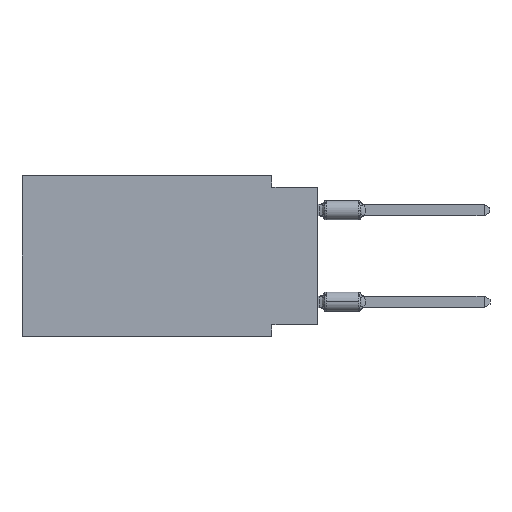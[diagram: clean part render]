
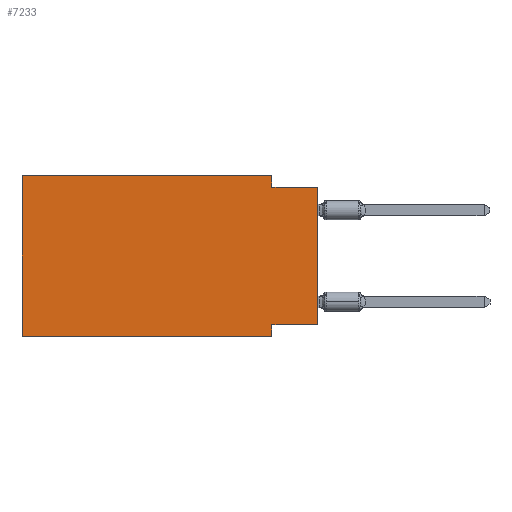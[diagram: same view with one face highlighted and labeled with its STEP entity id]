
A CAD part, left-side view. The second image highlights one B-rep face of the part: STEP entity #7233.
In plain terms, the highlighted planar face has unit normal (-1, 0, 0).
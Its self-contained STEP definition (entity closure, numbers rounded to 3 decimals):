
#296 = LINE ( 'NONE', #4620, #5544 ) ;
#353 = VECTOR ( 'NONE', #8296, 1000. ) ;
#519 = DIRECTION ( 'NONE',  ( 0., 0., -1. ) ) ;
#1118 = VECTOR ( 'NONE', #7778, 1000. ) ;
#1343 = CARTESIAN_POINT ( 'NONE',  ( 0., 16.383, 0. ) ) ;
#1543 = LINE ( 'NONE', #9942, #6392 ) ;
#2007 = VERTEX_POINT ( 'NONE', #5867 ) ;
#2042 = VECTOR ( 'NONE', #11174, 1000. ) ;
#2226 = LINE ( 'NONE', #13601, #12030 ) ;
#2514 = CARTESIAN_POINT ( 'NONE',  ( 0., 2.54, 0. ) ) ;
#2855 = LINE ( 'NONE', #3956, #353 ) ;
#3309 = EDGE_CURVE ( 'NONE', #2007, #12671, #7925, .T. ) ;
#3340 = CARTESIAN_POINT ( 'NONE',  ( 0., 0., -0.635 ) ) ;
#3508 = CARTESIAN_POINT ( 'NONE',  ( 0., 16.383, 0. ) ) ;
#3920 = ORIENTED_EDGE ( 'NONE', *, *, #8619, .F. ) ;
#3956 = CARTESIAN_POINT ( 'NONE',  ( 0., 2.54, 0. ) ) ;
#4610 = DIRECTION ( 'NONE',  ( 0., 0., 1. ) ) ;
#4620 = CARTESIAN_POINT ( 'NONE',  ( 0., 16.383, 0. ) ) ;
#4792 = EDGE_CURVE ( 'NONE', #8683, #11143, #296, .T. ) ;
#5430 = VERTEX_POINT ( 'NONE', #5609 ) ;
#5544 = VECTOR ( 'NONE', #12830, 1000. ) ;
#5609 = CARTESIAN_POINT ( 'NONE',  ( 0., 2.54, -8.255 ) ) ;
#5702 = LINE ( 'NONE', #3508, #5746 ) ;
#5746 = VECTOR ( 'NONE', #4610, 1000. ) ;
#5867 = CARTESIAN_POINT ( 'NONE',  ( 0., 0., -8.255 ) ) ;
#5999 = VERTEX_POINT ( 'NONE', #11868 ) ;
#6045 = ORIENTED_EDGE ( 'NONE', *, *, #11906, .F. ) ;
#6241 = ORIENTED_EDGE ( 'NONE', *, *, #3309, .T. ) ;
#6392 = VECTOR ( 'NONE', #519, 1000. ) ;
#6410 = DIRECTION ( 'NONE',  ( 0., 1., 0. ) ) ;
#6946 = EDGE_CURVE ( 'NONE', #11143, #5999, #2855, .T. ) ;
#7233 = ADVANCED_FACE ( 'NONE', ( #10013 ), #7601, .F. ) ;
#7494 = CARTESIAN_POINT ( 'NONE',  ( 0., 16.383, -8.89 ) ) ;
#7601 = PLANE ( 'NONE',  #8258 ) ;
#7654 = CARTESIAN_POINT ( 'NONE',  ( 0., 16.383, 0. ) ) ;
#7778 = DIRECTION ( 'NONE',  ( 0., -1., 0. ) ) ;
#7925 = LINE ( 'NONE', #12210, #2042 ) ;
#7982 = CARTESIAN_POINT ( 'NONE',  ( 0., 0., -0.635 ) ) ;
#8111 = DIRECTION ( 'NONE',  ( 0., -1., 0. ) ) ;
#8258 = AXIS2_PLACEMENT_3D ( 'NONE', #1343, #9876, #10774 ) ;
#8296 = DIRECTION ( 'NONE',  ( 0., 0., -1. ) ) ;
#8545 = CARTESIAN_POINT ( 'NONE',  ( 0., 2.54, -8.89 ) ) ;
#8619 = EDGE_CURVE ( 'NONE', #2007, #5430, #2226, .T. ) ;
#8683 = VERTEX_POINT ( 'NONE', #7654 ) ;
#9019 = ORIENTED_EDGE ( 'NONE', *, *, #11236, .F. ) ;
#9079 = VECTOR ( 'NONE', #8111, 1000. ) ;
#9876 = DIRECTION ( 'NONE',  ( 1., 0., 0. ) ) ;
#9920 = ORIENTED_EDGE ( 'NONE', *, *, #4792, .F. ) ;
#9942 = CARTESIAN_POINT ( 'NONE',  ( 0., 2.54, -8.89 ) ) ;
#10013 = FACE_OUTER_BOUND ( 'NONE', #12195, .T. ) ;
#10774 = DIRECTION ( 'NONE',  ( 0., 0., -1. ) ) ;
#10805 = EDGE_CURVE ( 'NONE', #11898, #11459, #11007, .T. ) ;
#11007 = LINE ( 'NONE', #13092, #1118 ) ;
#11143 = VERTEX_POINT ( 'NONE', #2514 ) ;
#11174 = DIRECTION ( 'NONE',  ( 0., 0., 1. ) ) ;
#11236 = EDGE_CURVE ( 'NONE', #5430, #11459, #1543, .T. ) ;
#11459 = VERTEX_POINT ( 'NONE', #8545 ) ;
#11613 = ORIENTED_EDGE ( 'NONE', *, *, #6946, .F. ) ;
#11837 = ORIENTED_EDGE ( 'NONE', *, *, #10805, .T. ) ;
#11868 = CARTESIAN_POINT ( 'NONE',  ( 0., 2.54, -0.635 ) ) ;
#11898 = VERTEX_POINT ( 'NONE', #7494 ) ;
#11906 = EDGE_CURVE ( 'NONE', #11898, #8683, #5702, .T. ) ;
#12030 = VECTOR ( 'NONE', #6410, 1000. ) ;
#12051 = LINE ( 'NONE', #7982, #9079 ) ;
#12099 = ORIENTED_EDGE ( 'NONE', *, *, #13152, .F. ) ;
#12195 = EDGE_LOOP ( 'NONE', ( #6241, #12099, #11613, #9920, #6045, #11837, #9019, #3920 ) ) ;
#12210 = CARTESIAN_POINT ( 'NONE',  ( 0., 0., 0. ) ) ;
#12671 = VERTEX_POINT ( 'NONE', #3340 ) ;
#12830 = DIRECTION ( 'NONE',  ( 0., -1., 0. ) ) ;
#13092 = CARTESIAN_POINT ( 'NONE',  ( 0., 16.383, -8.89 ) ) ;
#13152 = EDGE_CURVE ( 'NONE', #5999, #12671, #12051, .T. ) ;
#13601 = CARTESIAN_POINT ( 'NONE',  ( 0., 0., -8.255 ) ) ;
